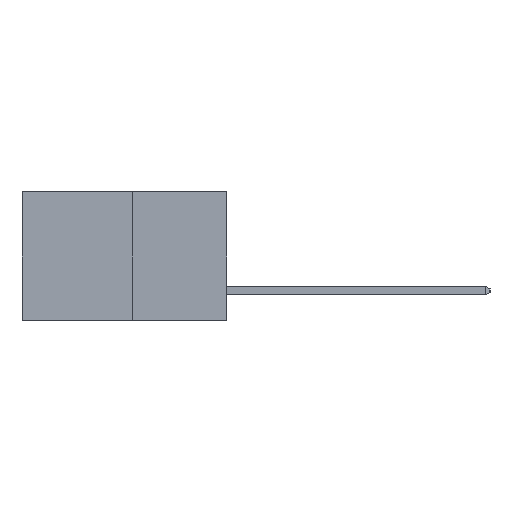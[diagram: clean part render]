
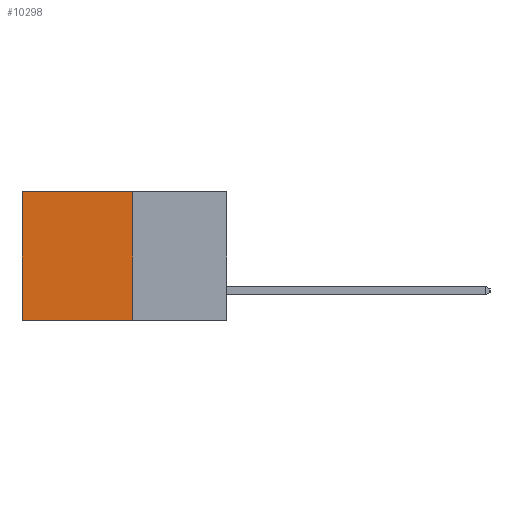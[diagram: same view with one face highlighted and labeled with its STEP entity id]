
A CAD part, left-side view. The second image highlights one B-rep face of the part: STEP entity #10298.
In plain terms, the highlighted planar face has unit normal (-1, 0, 0).
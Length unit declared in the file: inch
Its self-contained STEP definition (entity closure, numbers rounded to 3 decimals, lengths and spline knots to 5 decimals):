
#505 = EDGE_LOOP ( 'NONE', ( #1944, #4004, #1669, #5885 ) ) ;
#613 = DIRECTION ( 'NONE',  ( 0., 0., -1. ) ) ;
#1046 = EDGE_CURVE ( 'NONE', #1644, #3178, #4807, .T. ) ;
#1644 = VERTEX_POINT ( 'NONE', #3521 ) ;
#1654 = PLANE ( 'NONE',  #8261 ) ;
#1669 = ORIENTED_EDGE ( 'NONE', *, *, #4121, .F. ) ;
#1944 = ORIENTED_EDGE ( 'NONE', *, *, #8460, .T. ) ;
#2482 = EDGE_CURVE ( 'NONE', #2988, #3155, #4430, .T. ) ;
#2564 = VECTOR ( 'NONE', #4858, 39.37008 ) ;
#2988 = VERTEX_POINT ( 'NONE', #5745 ) ;
#3032 = CARTESIAN_POINT ( 'NONE',  ( 0.277, 0.27, -0.37 ) ) ;
#3155 = VERTEX_POINT ( 'NONE', #7700 ) ;
#3178 = VERTEX_POINT ( 'NONE', #3441 ) ;
#3433 = DIRECTION ( 'NONE',  ( 1., 0., 0. ) ) ;
#3441 = CARTESIAN_POINT ( 'NONE',  ( 0.277, 0.59, 0. ) ) ;
#3521 = CARTESIAN_POINT ( 'NONE',  ( 0.277, 0.27, 0. ) ) ;
#4004 = ORIENTED_EDGE ( 'NONE', *, *, #2482, .F. ) ;
#4121 = EDGE_CURVE ( 'NONE', #1644, #2988, #6018, .T. ) ;
#4430 = LINE ( 'NONE', #3032, #10354 ) ;
#4807 = LINE ( 'NONE', #5739, #6934 ) ;
#4851 = CARTESIAN_POINT ( 'NONE',  ( 0.277, 0.59, -0.37 ) ) ;
#4858 = DIRECTION ( 'NONE',  ( 0., 0., -1. ) ) ;
#5128 = FACE_OUTER_BOUND ( 'NONE', #505, .T. ) ;
#5464 = DIRECTION ( 'NONE',  ( 0., 1., 0. ) ) ;
#5739 = CARTESIAN_POINT ( 'NONE',  ( 0.277, 0.27, 0. ) ) ;
#5745 = CARTESIAN_POINT ( 'NONE',  ( 0.277, 0.27, -0.37 ) ) ;
#5885 = ORIENTED_EDGE ( 'NONE', *, *, #1046, .T. ) ;
#6018 = LINE ( 'NONE', #9242, #9870 ) ;
#6934 = VECTOR ( 'NONE', #5464, 39.37008 ) ;
#7158 = LINE ( 'NONE', #4851, #2564 ) ;
#7423 = CARTESIAN_POINT ( 'NONE',  ( 0.277, 0.27, -0.37 ) ) ;
#7700 = CARTESIAN_POINT ( 'NONE',  ( 0.277, 0.59, -0.37 ) ) ;
#8261 = AXIS2_PLACEMENT_3D ( 'NONE', #7423, #3433, #8971 ) ;
#8460 = EDGE_CURVE ( 'NONE', #3178, #3155, #7158, .T. ) ;
#8945 = DIRECTION ( 'NONE',  ( 0., 1., 0. ) ) ;
#8971 = DIRECTION ( 'NONE',  ( 0., 0., -1. ) ) ;
#9242 = CARTESIAN_POINT ( 'NONE',  ( 0.277, 0.27, -0.37 ) ) ;
#9870 = VECTOR ( 'NONE', #613, 39.37008 ) ;
#10298 = ADVANCED_FACE ( 'NONE', ( #5128 ), #1654, .F. ) ;
#10354 = VECTOR ( 'NONE', #8945, 39.37008 ) ;
